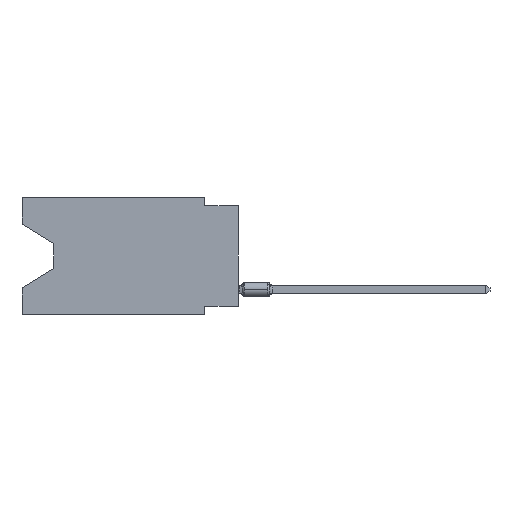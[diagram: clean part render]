
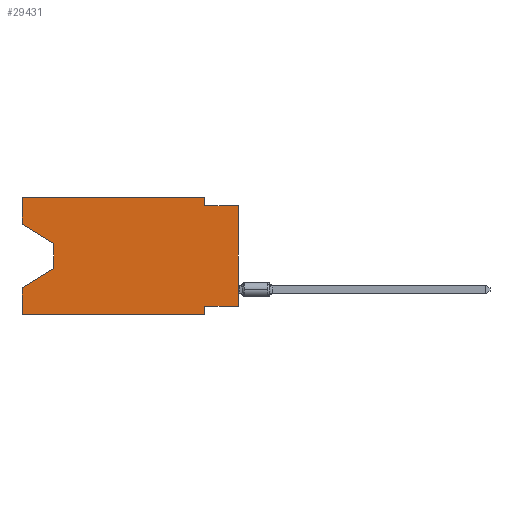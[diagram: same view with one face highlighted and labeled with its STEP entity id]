
A CAD part, left-side view. The second image highlights one B-rep face of the part: STEP entity #29431.
In plain terms, the highlighted planar face has unit normal (-1, 0, 0).
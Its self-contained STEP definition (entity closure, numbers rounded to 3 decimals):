
#438 = FACE_OUTER_BOUND ( 'NONE', #34541, .T. ) ;
#640 = CARTESIAN_POINT ( 'NONE',  ( 0., 2.54, -8.89 ) ) ;
#653 = VERTEX_POINT ( 'NONE', #640 ) ;
#1268 = ORIENTED_EDGE ( 'NONE', *, *, #23106, .T. ) ;
#1342 = VECTOR ( 'NONE', #2028, 1000. ) ;
#1618 = EDGE_CURVE ( 'NONE', #4633, #31873, #28967, .T. ) ;
#1961 = LINE ( 'NONE', #28373, #5310 ) ;
#2028 = DIRECTION ( 'NONE',  ( 0., 1., 0. ) ) ;
#2177 = VERTEX_POINT ( 'NONE', #29870 ) ;
#2198 = CARTESIAN_POINT ( 'NONE',  ( 0., 2.54, 0. ) ) ;
#3124 = VERTEX_POINT ( 'NONE', #21513 ) ;
#3614 = DIRECTION ( 'NONE',  ( 0., 0.855, -0.519 ) ) ;
#4067 = VECTOR ( 'NONE', #3614, 1000. ) ;
#4237 = EDGE_CURVE ( 'NONE', #4633, #653, #32671, .T. ) ;
#4473 = VERTEX_POINT ( 'NONE', #25600 ) ;
#4633 = VERTEX_POINT ( 'NONE', #28994 ) ;
#5063 = LINE ( 'NONE', #16667, #30808 ) ;
#5219 = CARTESIAN_POINT ( 'NONE',  ( 0., 2.54, -8.255 ) ) ;
#5310 = VECTOR ( 'NONE', #13576, 1000. ) ;
#5451 = LINE ( 'NONE', #37011, #1342 ) ;
#5809 = ORIENTED_EDGE ( 'NONE', *, *, #10195, .T. ) ;
#6265 = DIRECTION ( 'NONE',  ( 0., -1., 0. ) ) ;
#6699 = DIRECTION ( 'NONE',  ( 0., 0., -1. ) ) ;
#6705 = EDGE_CURVE ( 'NONE', #32779, #36834, #5451, .T. ) ;
#7086 = EDGE_CURVE ( 'NONE', #2177, #3124, #14489, .T. ) ;
#7432 = LINE ( 'NONE', #13525, #37440 ) ;
#8794 = ORIENTED_EDGE ( 'NONE', *, *, #11689, .F. ) ;
#8986 = VECTOR ( 'NONE', #6265, 1000. ) ;
#9195 = CARTESIAN_POINT ( 'NONE',  ( 0., 16.383, 0. ) ) ;
#10195 = EDGE_CURVE ( 'NONE', #4473, #31873, #20936, .T. ) ;
#10581 = LINE ( 'NONE', #2198, #31718 ) ;
#11296 = ORIENTED_EDGE ( 'NONE', *, *, #7086, .F. ) ;
#11689 = EDGE_CURVE ( 'NONE', #34348, #27493, #12304, .T. ) ;
#12041 = PLANE ( 'NONE',  #29034 ) ;
#12258 = EDGE_CURVE ( 'NONE', #22199, #34348, #5063, .T. ) ;
#12304 = LINE ( 'NONE', #32812, #24124 ) ;
#13116 = VECTOR ( 'NONE', #25525, 1000. ) ;
#13525 = CARTESIAN_POINT ( 'NONE',  ( 0., 0., 0. ) ) ;
#13576 = DIRECTION ( 'NONE',  ( 0., -0.855, -0.519 ) ) ;
#14489 = LINE ( 'NONE', #31066, #30317 ) ;
#14595 = VECTOR ( 'NONE', #23291, 1000. ) ;
#14658 = CARTESIAN_POINT ( 'NONE',  ( 0., 13.97, -5.385 ) ) ;
#14854 = CARTESIAN_POINT ( 'NONE',  ( 0., 16.383, -2.038 ) ) ;
#14932 = ORIENTED_EDGE ( 'NONE', *, *, #4237, .T. ) ;
#14952 = CARTESIAN_POINT ( 'NONE',  ( 0., 13.97, -3.505 ) ) ;
#16667 = CARTESIAN_POINT ( 'NONE',  ( 0., 16.383, 0. ) ) ;
#18061 = CARTESIAN_POINT ( 'NONE',  ( 0., 16.383, -8.89 ) ) ;
#18594 = ORIENTED_EDGE ( 'NONE', *, *, #28374, .T. ) ;
#19460 = CARTESIAN_POINT ( 'NONE',  ( 0., 2.54, -8.89 ) ) ;
#20023 = CARTESIAN_POINT ( 'NONE',  ( 0., 2.54, 0. ) ) ;
#20195 = DIRECTION ( 'NONE',  ( 0., -1., 0. ) ) ;
#20366 = EDGE_CURVE ( 'NONE', #27493, #2177, #10581, .T. ) ;
#20658 = LINE ( 'NONE', #14952, #37049 ) ;
#20687 = ORIENTED_EDGE ( 'NONE', *, *, #20366, .F. ) ;
#20936 = LINE ( 'NONE', #14658, #4067 ) ;
#21513 = CARTESIAN_POINT ( 'NONE',  ( 0., 0., -0.635 ) ) ;
#22186 = DIRECTION ( 'NONE',  ( 0., 0., -1. ) ) ;
#22199 = VERTEX_POINT ( 'NONE', #14854 ) ;
#23106 = EDGE_CURVE ( 'NONE', #37329, #4473, #20658, .T. ) ;
#23291 = DIRECTION ( 'NONE',  ( 0., 0., 1. ) ) ;
#24084 = ORIENTED_EDGE ( 'NONE', *, *, #12258, .F. ) ;
#24124 = VECTOR ( 'NONE', #29572, 1000. ) ;
#24555 = DIRECTION ( 'NONE',  ( 0., 0., 1. ) ) ;
#25525 = DIRECTION ( 'NONE',  ( 0., 0., -1. ) ) ;
#25535 = CARTESIAN_POINT ( 'NONE',  ( 0., 16.383, -6.852 ) ) ;
#25558 = ORIENTED_EDGE ( 'NONE', *, *, #6705, .F. ) ;
#25600 = CARTESIAN_POINT ( 'NONE',  ( 0., 13.97, -5.385 ) ) ;
#26467 = CARTESIAN_POINT ( 'NONE',  ( 0., 13.97, -3.505 ) ) ;
#27493 = VERTEX_POINT ( 'NONE', #20023 ) ;
#27652 = EDGE_CURVE ( 'NONE', #32779, #3124, #7432, .T. ) ;
#28373 = CARTESIAN_POINT ( 'NONE',  ( 0., 16.383, -2.038 ) ) ;
#28374 = EDGE_CURVE ( 'NONE', #22199, #37329, #1961, .T. ) ;
#28967 = LINE ( 'NONE', #29163, #14595 ) ;
#28994 = CARTESIAN_POINT ( 'NONE',  ( 0., 16.383, -8.89 ) ) ;
#29034 = AXIS2_PLACEMENT_3D ( 'NONE', #9195, #32745, #6699 ) ;
#29163 = CARTESIAN_POINT ( 'NONE',  ( 0., 16.383, 0. ) ) ;
#29431 = ADVANCED_FACE ( 'NONE', ( #438 ), #12041, .F. ) ;
#29572 = DIRECTION ( 'NONE',  ( 0., -1., 0. ) ) ;
#29870 = CARTESIAN_POINT ( 'NONE',  ( 0., 2.54, -0.635 ) ) ;
#30317 = VECTOR ( 'NONE', #20195, 1000. ) ;
#30808 = VECTOR ( 'NONE', #36615, 1000. ) ;
#31066 = CARTESIAN_POINT ( 'NONE',  ( 0., 0., -0.635 ) ) ;
#31718 = VECTOR ( 'NONE', #22186, 1000. ) ;
#31873 = VERTEX_POINT ( 'NONE', #25535 ) ;
#32671 = LINE ( 'NONE', #18061, #8986 ) ;
#32745 = DIRECTION ( 'NONE',  ( 1., 0., 0. ) ) ;
#32779 = VERTEX_POINT ( 'NONE', #35281 ) ;
#32812 = CARTESIAN_POINT ( 'NONE',  ( 0., 16.383, 0. ) ) ;
#32830 = ORIENTED_EDGE ( 'NONE', *, *, #27652, .T. ) ;
#34348 = VERTEX_POINT ( 'NONE', #35654 ) ;
#34541 = EDGE_LOOP ( 'NONE', ( #18594, #1268, #5809, #35300, #14932, #34691, #25558, #32830, #11296, #20687, #8794, #24084 ) ) ;
#34691 = ORIENTED_EDGE ( 'NONE', *, *, #37169, .F. ) ;
#35281 = CARTESIAN_POINT ( 'NONE',  ( 0., 0., -8.255 ) ) ;
#35300 = ORIENTED_EDGE ( 'NONE', *, *, #1618, .F. ) ;
#35466 = DIRECTION ( 'NONE',  ( 0., 0., -1. ) ) ;
#35654 = CARTESIAN_POINT ( 'NONE',  ( 0., 16.383, 0. ) ) ;
#36615 = DIRECTION ( 'NONE',  ( 0., 0., 1. ) ) ;
#36834 = VERTEX_POINT ( 'NONE', #5219 ) ;
#36927 = LINE ( 'NONE', #19460, #13116 ) ;
#37011 = CARTESIAN_POINT ( 'NONE',  ( 0., 0., -8.255 ) ) ;
#37049 = VECTOR ( 'NONE', #35466, 1000. ) ;
#37169 = EDGE_CURVE ( 'NONE', #36834, #653, #36927, .T. ) ;
#37329 = VERTEX_POINT ( 'NONE', #26467 ) ;
#37440 = VECTOR ( 'NONE', #24555, 1000. ) ;
